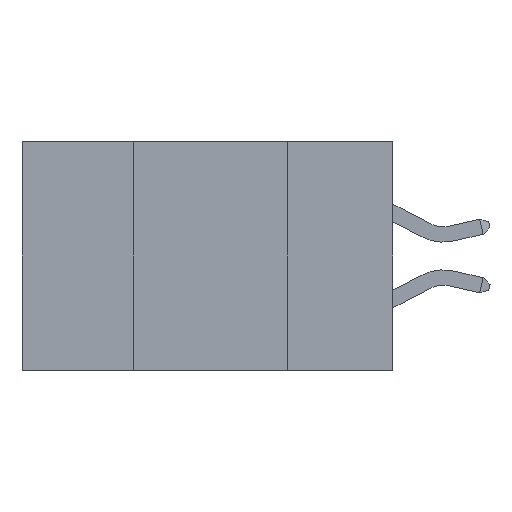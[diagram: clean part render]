
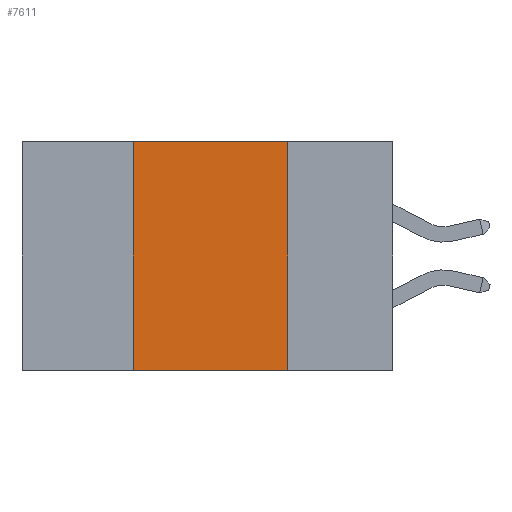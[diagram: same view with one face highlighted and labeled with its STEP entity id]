
A CAD part, left-side view. The second image highlights one B-rep face of the part: STEP entity #7611.
In plain terms, the highlighted planar face has unit normal (-1, 0, 0).
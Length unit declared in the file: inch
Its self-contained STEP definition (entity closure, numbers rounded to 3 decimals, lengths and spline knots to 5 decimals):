
#511 = CARTESIAN_POINT ( 'NONE',  ( 0., 0.6, 0. ) ) ;
#1161 = ORIENTED_EDGE ( 'NONE', *, *, #10557, .F. ) ;
#1177 = VECTOR ( 'NONE', #4635, 39.37008 ) ;
#1966 = DIRECTION ( 'NONE',  ( 0., 0., -1. ) ) ;
#2813 = EDGE_CURVE ( 'NONE', #4094, #5766, #14252, .T. ) ;
#2824 = LINE ( 'NONE', #15823, #16854 ) ;
#3387 = VECTOR ( 'NONE', #16689, 39.37008 ) ;
#3408 = CARTESIAN_POINT ( 'NONE',  ( 0., 0.17, 0. ) ) ;
#3680 = DIRECTION ( 'NONE',  ( 0., 0., -1. ) ) ;
#3731 = ORIENTED_EDGE ( 'NONE', *, *, #2813, .F. ) ;
#4094 = VERTEX_POINT ( 'NONE', #15997 ) ;
#4635 = DIRECTION ( 'NONE',  ( 0., -1., 0. ) ) ;
#5025 = LINE ( 'NONE', #7343, #1177 ) ;
#5766 = VERTEX_POINT ( 'NONE', #13866 ) ;
#6951 = FACE_OUTER_BOUND ( 'NONE', #7091, .T. ) ;
#7091 = EDGE_LOOP ( 'NONE', ( #1161, #8549, #3731, #7154 ) ) ;
#7154 = ORIENTED_EDGE ( 'NONE', *, *, #7505, .T. ) ;
#7343 = CARTESIAN_POINT ( 'NONE',  ( 0., 0.6, -0.37 ) ) ;
#7505 = EDGE_CURVE ( 'NONE', #4094, #8587, #5025, .T. ) ;
#7611 = ADVANCED_FACE ( 'NONE', ( #6951 ), #15607, .F. ) ;
#8277 = LINE ( 'NONE', #8381, #11423 ) ;
#8381 = CARTESIAN_POINT ( 'NONE',  ( 0., 0.6, 0. ) ) ;
#8549 = ORIENTED_EDGE ( 'NONE', *, *, #11469, .F. ) ;
#8587 = VERTEX_POINT ( 'NONE', #13619 ) ;
#10292 = DIRECTION ( 'NONE',  ( 1., 0., 0. ) ) ;
#10557 = EDGE_CURVE ( 'NONE', #17012, #8587, #2824, .T. ) ;
#11423 = VECTOR ( 'NONE', #17694, 39.37008 ) ;
#11469 = EDGE_CURVE ( 'NONE', #5766, #17012, #8277, .T. ) ;
#13619 = CARTESIAN_POINT ( 'NONE',  ( 0., 0.17, -0.37 ) ) ;
#13866 = CARTESIAN_POINT ( 'NONE',  ( 0., 0.42, 0. ) ) ;
#14252 = LINE ( 'NONE', #16994, #3387 ) ;
#15607 = PLANE ( 'NONE',  #17369 ) ;
#15823 = CARTESIAN_POINT ( 'NONE',  ( 0., 0.17, 0. ) ) ;
#15997 = CARTESIAN_POINT ( 'NONE',  ( 0., 0.42, -0.37 ) ) ;
#16689 = DIRECTION ( 'NONE',  ( 0., 0., 1. ) ) ;
#16854 = VECTOR ( 'NONE', #3680, 39.37008 ) ;
#16994 = CARTESIAN_POINT ( 'NONE',  ( 0., 0.42, 0. ) ) ;
#17012 = VERTEX_POINT ( 'NONE', #3408 ) ;
#17369 = AXIS2_PLACEMENT_3D ( 'NONE', #511, #10292, #1966 ) ;
#17694 = DIRECTION ( 'NONE',  ( 0., -1., 0. ) ) ;
